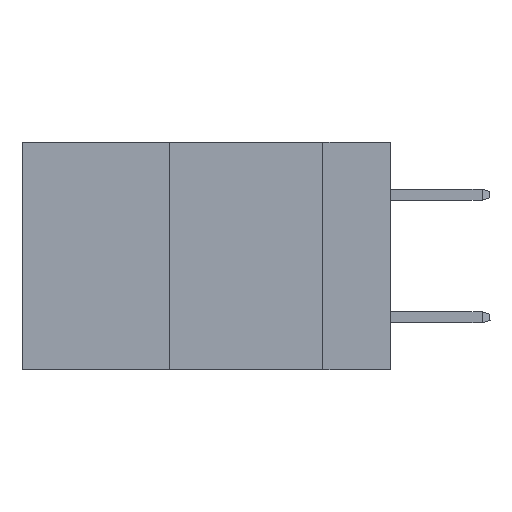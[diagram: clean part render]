
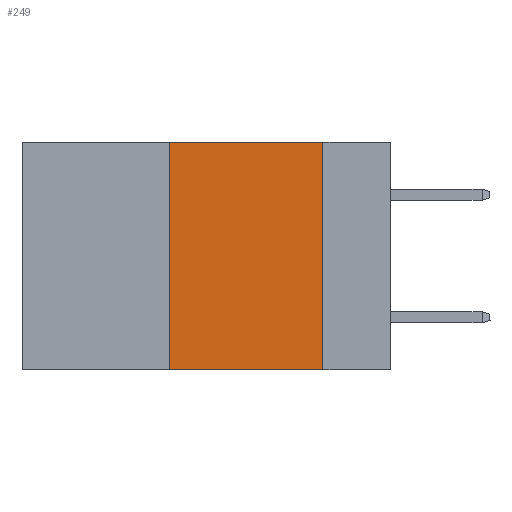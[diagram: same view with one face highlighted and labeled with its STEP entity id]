
A CAD part, left-side view. The second image highlights one B-rep face of the part: STEP entity #249.
In plain terms, the highlighted planar face has unit normal (-1, 0, 0).
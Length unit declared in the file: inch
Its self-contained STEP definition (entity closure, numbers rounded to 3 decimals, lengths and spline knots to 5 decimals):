
#138 = VECTOR ( 'NONE', #11344, 39.37008 ) ;
#249 = ADVANCED_FACE ( 'NONE', ( #3385 ), #7464, .F. ) ;
#375 = LINE ( 'NONE', #5128, #8429 ) ;
#801 = VERTEX_POINT ( 'NONE', #5686 ) ;
#1403 = VERTEX_POINT ( 'NONE', #10175 ) ;
#2332 = ORIENTED_EDGE ( 'NONE', *, *, #8206, .T. ) ;
#2551 = EDGE_CURVE ( 'NONE', #9784, #801, #4517, .T. ) ;
#3148 = CARTESIAN_POINT ( 'NONE',  ( 0., 0.36, -0.37 ) ) ;
#3192 = EDGE_CURVE ( 'NONE', #7869, #1403, #10382, .T. ) ;
#3385 = FACE_OUTER_BOUND ( 'NONE', #9749, .T. ) ;
#3555 = ORIENTED_EDGE ( 'NONE', *, *, #4709, .F. ) ;
#4083 = VECTOR ( 'NONE', #6567, 39.37008 ) ;
#4517 = LINE ( 'NONE', #10379, #11612 ) ;
#4709 = EDGE_CURVE ( 'NONE', #1403, #9784, #375, .T. ) ;
#4821 = DIRECTION ( 'NONE',  ( 0., 0., -1. ) ) ;
#5128 = CARTESIAN_POINT ( 'NONE',  ( 0., 0.6, 0. ) ) ;
#5686 = CARTESIAN_POINT ( 'NONE',  ( 0., 0.11, -0.37 ) ) ;
#5808 = CARTESIAN_POINT ( 'NONE',  ( 0., 0.36, 0. ) ) ;
#6076 = AXIS2_PLACEMENT_3D ( 'NONE', #10474, #10537, #4821 ) ;
#6567 = DIRECTION ( 'NONE',  ( 0., -1., 0. ) ) ;
#7464 = PLANE ( 'NONE',  #6076 ) ;
#7869 = VERTEX_POINT ( 'NONE', #3148 ) ;
#8206 = EDGE_CURVE ( 'NONE', #7869, #801, #11758, .T. ) ;
#8400 = ORIENTED_EDGE ( 'NONE', *, *, #3192, .F. ) ;
#8429 = VECTOR ( 'NONE', #10726, 39.37008 ) ;
#9335 = CARTESIAN_POINT ( 'NONE',  ( 0., 0.6, -0.37 ) ) ;
#9450 = ORIENTED_EDGE ( 'NONE', *, *, #2551, .F. ) ;
#9749 = EDGE_LOOP ( 'NONE', ( #9450, #3555, #8400, #2332 ) ) ;
#9784 = VERTEX_POINT ( 'NONE', #9885 ) ;
#9885 = CARTESIAN_POINT ( 'NONE',  ( 0., 0.11, 0. ) ) ;
#10175 = CARTESIAN_POINT ( 'NONE',  ( 0., 0.36, 0. ) ) ;
#10379 = CARTESIAN_POINT ( 'NONE',  ( 0., 0.11, 0. ) ) ;
#10382 = LINE ( 'NONE', #5808, #138 ) ;
#10474 = CARTESIAN_POINT ( 'NONE',  ( 0., 0.6, 0. ) ) ;
#10537 = DIRECTION ( 'NONE',  ( 1., 0., 0. ) ) ;
#10726 = DIRECTION ( 'NONE',  ( 0., -1., 0. ) ) ;
#11241 = DIRECTION ( 'NONE',  ( 0., 0., -1. ) ) ;
#11344 = DIRECTION ( 'NONE',  ( 0., 0., 1. ) ) ;
#11612 = VECTOR ( 'NONE', #11241, 39.37008 ) ;
#11758 = LINE ( 'NONE', #9335, #4083 ) ;
